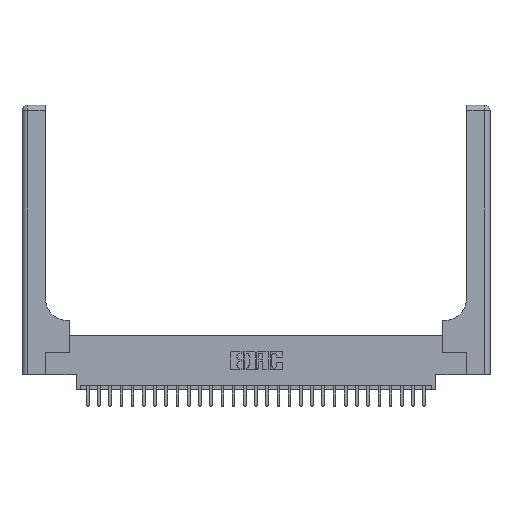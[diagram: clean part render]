
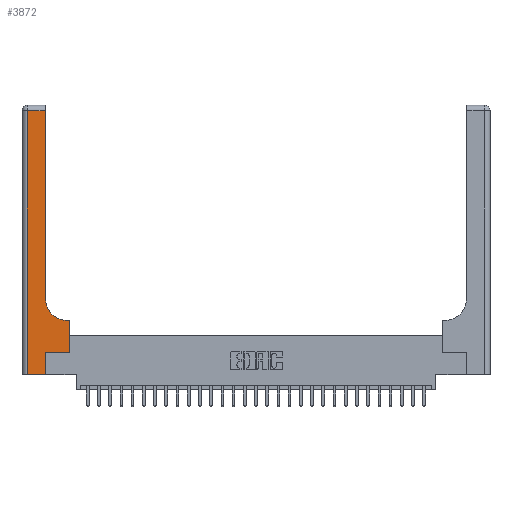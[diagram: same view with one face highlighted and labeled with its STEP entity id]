
A CAD part, top view. The second image highlights one B-rep face of the part: STEP entity #3872.
In plain terms, the highlighted planar face has unit normal (0, 0, 1).
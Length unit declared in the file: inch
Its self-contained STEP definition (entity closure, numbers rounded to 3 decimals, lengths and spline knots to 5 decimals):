
#513 = DIRECTION ( 'NONE',  ( -1., 0., 0. ) ) ;
#814 = CARTESIAN_POINT ( 'NONE',  ( 0.26, 0.6, 0.37 ) ) ;
#1394 = CARTESIAN_POINT ( 'NONE',  ( 0.06, 0., 0.37 ) ) ;
#1421 = DIRECTION ( 'NONE',  ( 1., 0., 0. ) ) ;
#1726 = ORIENTED_EDGE ( 'NONE', *, *, #17356, .T. ) ;
#1855 = DIRECTION ( 'NONE',  ( 0., 1., 0. ) ) ;
#2670 = EDGE_CURVE ( 'NONE', #22446, #17381, #13819, .T. ) ;
#3872 = ADVANCED_FACE ( 'NONE', ( #18782 ), #23171, .F. ) ;
#4369 = VECTOR ( 'NONE', #13176, 39.37008 ) ;
#4824 = CARTESIAN_POINT ( 'NONE',  ( 0.528, 0.6, 0.37 ) ) ;
#5082 = AXIS2_PLACEMENT_3D ( 'NONE', #19012, #10538, #25192 ) ;
#5487 = VERTEX_POINT ( 'NONE', #23991 ) ;
#6382 = ORIENTED_EDGE ( 'NONE', *, *, #2670, .T. ) ;
#6968 = CARTESIAN_POINT ( 'NONE',  ( 0.51, 0.85, 0.37 ) ) ;
#7074 = VECTOR ( 'NONE', #24130, 39.37008 ) ;
#7846 = EDGE_CURVE ( 'NONE', #22155, #22446, #20125, .T. ) ;
#8049 = VERTEX_POINT ( 'NONE', #9706 ) ;
#8222 = VECTOR ( 'NONE', #1855, 39.37008 ) ;
#8295 = CARTESIAN_POINT ( 'NONE',  ( 0.265, 0., 0.37 ) ) ;
#8418 = LINE ( 'NONE', #17981, #7074 ) ;
#8732 = VERTEX_POINT ( 'NONE', #18686 ) ;
#8986 = DIRECTION ( 'NONE',  ( 0., 1., 0. ) ) ;
#9109 = DIRECTION ( 'NONE',  ( 1., 0., 0. ) ) ;
#9147 = ORIENTED_EDGE ( 'NONE', *, *, #20562, .T. ) ;
#9706 = CARTESIAN_POINT ( 'NONE',  ( 0.06, 2.94, 0.37 ) ) ;
#10287 = EDGE_CURVE ( 'NONE', #24091, #8049, #8418, .T. ) ;
#10538 = DIRECTION ( 'NONE',  ( 0., 0., -1. ) ) ;
#11811 = ORIENTED_EDGE ( 'NONE', *, *, #14774, .T. ) ;
#12101 = CARTESIAN_POINT ( 'NONE',  ( 0.51, 0.6, 0.37 ) ) ;
#13176 = DIRECTION ( 'NONE',  ( 0., 1., 0. ) ) ;
#13819 = LINE ( 'NONE', #814, #18801 ) ;
#13857 = LINE ( 'NONE', #8295, #8222 ) ;
#13946 = CARTESIAN_POINT ( 'NONE',  ( 0.528, 0.25, 0.37 ) ) ;
#14420 = AXIS2_PLACEMENT_3D ( 'NONE', #6968, #21766, #9109 ) ;
#14432 = EDGE_CURVE ( 'NONE', #17381, #21041, #16362, .T. ) ;
#14708 = ORIENTED_EDGE ( 'NONE', *, *, #7846, .T. ) ;
#14774 = EDGE_CURVE ( 'NONE', #8049, #18282, #15352, .T. ) ;
#14775 = ORIENTED_EDGE ( 'NONE', *, *, #10287, .T. ) ;
#15219 = EDGE_LOOP ( 'NONE', ( #9147, #14775, #11811, #20462, #23740, #1726, #14708, #6382, #23424 ) ) ;
#15352 = LINE ( 'NONE', #26448, #25091 ) ;
#16316 = CARTESIAN_POINT ( 'NONE',  ( 0.265, 0.25, 0.37 ) ) ;
#16362 = CIRCLE ( 'NONE', #14420, 0.25 ) ;
#16593 = VECTOR ( 'NONE', #1421, 39.37008 ) ;
#17356 = EDGE_CURVE ( 'NONE', #5487, #22155, #22797, .T. ) ;
#17381 = VERTEX_POINT ( 'NONE', #12101 ) ;
#17440 = CARTESIAN_POINT ( 'NONE',  ( 0.528, 0.25, 0.37 ) ) ;
#17981 = CARTESIAN_POINT ( 'NONE',  ( 0., 2.94, 0.37 ) ) ;
#18171 = CARTESIAN_POINT ( 'NONE',  ( 0.26, 2.94, 0.37 ) ) ;
#18282 = VERTEX_POINT ( 'NONE', #1394 ) ;
#18433 = EDGE_CURVE ( 'NONE', #8732, #5487, #13857, .T. ) ;
#18686 = CARTESIAN_POINT ( 'NONE',  ( 0.265, 0., 0.37 ) ) ;
#18782 = FACE_OUTER_BOUND ( 'NONE', #15219, .T. ) ;
#18801 = VECTOR ( 'NONE', #513, 39.37008 ) ;
#19012 = CARTESIAN_POINT ( 'NONE',  ( 0., 3., 0.37 ) ) ;
#19732 = LINE ( 'NONE', #20410, #24531 ) ;
#20125 = LINE ( 'NONE', #17440, #24276 ) ;
#20410 = CARTESIAN_POINT ( 'NONE',  ( 0., 0., 0.37 ) ) ;
#20462 = ORIENTED_EDGE ( 'NONE', *, *, #26657, .T. ) ;
#20487 = DIRECTION ( 'NONE',  ( 0., -1., 0. ) ) ;
#20562 = EDGE_CURVE ( 'NONE', #21041, #24091, #21277, .T. ) ;
#21021 = CARTESIAN_POINT ( 'NONE',  ( 0.26, 0.85, 0.37 ) ) ;
#21041 = VERTEX_POINT ( 'NONE', #21021 ) ;
#21277 = LINE ( 'NONE', #23652, #4369 ) ;
#21766 = DIRECTION ( 'NONE',  ( 0., 0., -1. ) ) ;
#22155 = VERTEX_POINT ( 'NONE', #13946 ) ;
#22446 = VERTEX_POINT ( 'NONE', #4824 ) ;
#22797 = LINE ( 'NONE', #16316, #16593 ) ;
#23171 = PLANE ( 'NONE',  #5082 ) ;
#23424 = ORIENTED_EDGE ( 'NONE', *, *, #14432, .T. ) ;
#23652 = CARTESIAN_POINT ( 'NONE',  ( 0.26, 3., 0.37 ) ) ;
#23740 = ORIENTED_EDGE ( 'NONE', *, *, #18433, .T. ) ;
#23991 = CARTESIAN_POINT ( 'NONE',  ( 0.265, 0.25, 0.37 ) ) ;
#24091 = VERTEX_POINT ( 'NONE', #18171 ) ;
#24130 = DIRECTION ( 'NONE',  ( -1., 0., 0. ) ) ;
#24276 = VECTOR ( 'NONE', #8986, 39.37008 ) ;
#24531 = VECTOR ( 'NONE', #26540, 39.37008 ) ;
#25091 = VECTOR ( 'NONE', #20487, 39.37008 ) ;
#25192 = DIRECTION ( 'NONE',  ( -1., 0., 0. ) ) ;
#26448 = CARTESIAN_POINT ( 'NONE',  ( 0.06, 3., 0.37 ) ) ;
#26540 = DIRECTION ( 'NONE',  ( 1., 0., 0. ) ) ;
#26657 = EDGE_CURVE ( 'NONE', #18282, #8732, #19732, .T. ) ;
